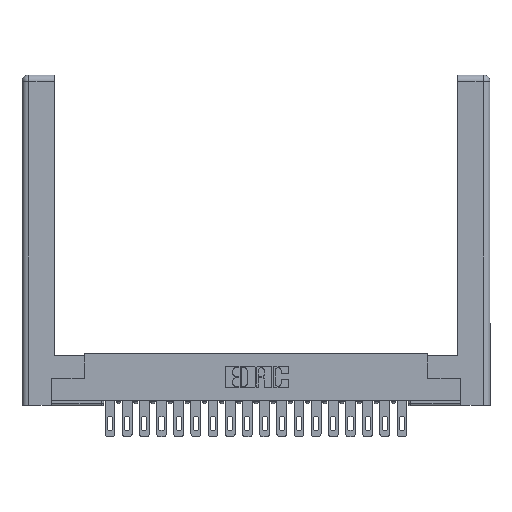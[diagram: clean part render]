
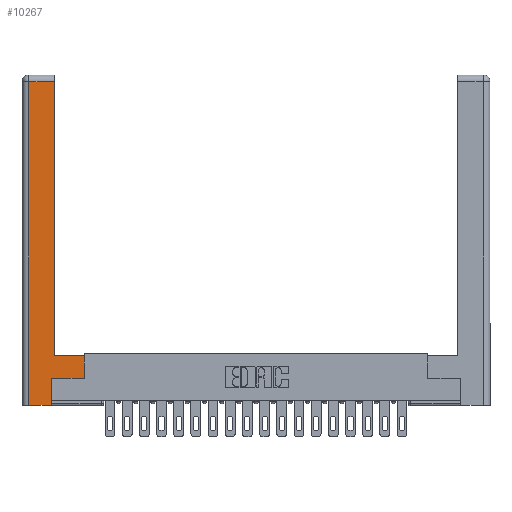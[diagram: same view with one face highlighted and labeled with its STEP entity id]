
A CAD part, top view. The second image highlights one B-rep face of the part: STEP entity #10267.
In plain terms, the highlighted planar face has unit normal (0, 0, 1).
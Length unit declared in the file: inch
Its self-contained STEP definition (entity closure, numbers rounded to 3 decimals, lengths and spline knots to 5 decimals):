
#67 = ORIENTED_EDGE ( 'NONE', *, *, #13105, .T. ) ;
#101 = ORIENTED_EDGE ( 'NONE', *, *, #14070, .T. ) ;
#666 = CARTESIAN_POINT ( 'NONE',  ( 0.565, 0.245, 0. ) ) ;
#947 = DIRECTION ( 'NONE',  ( 0., 1., 0. ) ) ;
#1088 = CARTESIAN_POINT ( 'NONE',  ( 0.265, 0.245, 0. ) ) ;
#1178 = VECTOR ( 'NONE', #18576, 39.37008 ) ;
#1301 = ORIENTED_EDGE ( 'NONE', *, *, #3292, .T. ) ;
#1410 = DIRECTION ( 'NONE',  ( 1., 0., 0. ) ) ;
#2432 = EDGE_CURVE ( 'NONE', #15426, #3903, #2820, .T. ) ;
#2820 = LINE ( 'NONE', #9255, #4693 ) ;
#3093 = PLANE ( 'NONE',  #21550 ) ;
#3292 = EDGE_CURVE ( 'NONE', #12812, #11096, #19490, .T. ) ;
#3414 = DIRECTION ( 'NONE',  ( -1., 0., 0. ) ) ;
#3785 = CARTESIAN_POINT ( 'NONE',  ( 0.565, 0.45, 0. ) ) ;
#3903 = VERTEX_POINT ( 'NONE', #18792 ) ;
#4213 = ORIENTED_EDGE ( 'NONE', *, *, #19601, .T. ) ;
#4693 = VECTOR ( 'NONE', #947, 39.37008 ) ;
#4699 = LINE ( 'NONE', #17998, #10013 ) ;
#4708 = VECTOR ( 'NONE', #21230, 39.37008 ) ;
#5031 = VECTOR ( 'NONE', #17765, 39.37008 ) ;
#5453 = DIRECTION ( 'NONE',  ( -1., 0., 0. ) ) ;
#6202 = VECTOR ( 'NONE', #12877, 39.37008 ) ;
#7429 = ORIENTED_EDGE ( 'NONE', *, *, #18138, .T. ) ;
#7685 = CARTESIAN_POINT ( 'NONE',  ( 0.0615, 0., 0. ) ) ;
#7697 = DIRECTION ( 'NONE',  ( 0., 1., 0. ) ) ;
#8512 = CARTESIAN_POINT ( 'NONE',  ( 0.0615, 2.94, 0. ) ) ;
#8569 = CARTESIAN_POINT ( 'NONE',  ( 0.0615, 0., 0. ) ) ;
#9255 = CARTESIAN_POINT ( 'NONE',  ( 0.295, 3., 0. ) ) ;
#9862 = CARTESIAN_POINT ( 'NONE',  ( 0.565, 0.45, 0. ) ) ;
#10013 = VECTOR ( 'NONE', #1410, 39.37008 ) ;
#10267 = ADVANCED_FACE ( 'NONE', ( #11577 ), #3093, .F. ) ;
#10383 = CARTESIAN_POINT ( 'NONE',  ( 0.265, 0., 0. ) ) ;
#10795 = EDGE_CURVE ( 'NONE', #20568, #20995, #4699, .T. ) ;
#10889 = CARTESIAN_POINT ( 'NONE',  ( 0.295, 0.45, 0. ) ) ;
#10947 = CARTESIAN_POINT ( 'NONE',  ( 0.565, 0.245, 0. ) ) ;
#11066 = EDGE_CURVE ( 'NONE', #11096, #15426, #19307, .T. ) ;
#11096 = VERTEX_POINT ( 'NONE', #3785 ) ;
#11476 = DIRECTION ( 'NONE',  ( 0., 0., -1. ) ) ;
#11577 = FACE_OUTER_BOUND ( 'NONE', #19947, .T. ) ;
#11805 = VECTOR ( 'NONE', #5453, 39.37008 ) ;
#12812 = VERTEX_POINT ( 'NONE', #10947 ) ;
#12877 = DIRECTION ( 'NONE',  ( 0., 1., 0. ) ) ;
#13105 = EDGE_CURVE ( 'NONE', #21238, #12812, #20766, .T. ) ;
#13149 = CARTESIAN_POINT ( 'NONE',  ( 0.0615, 2.94, 0. ) ) ;
#13505 = ORIENTED_EDGE ( 'NONE', *, *, #2432, .T. ) ;
#13707 = VERTEX_POINT ( 'NONE', #13149 ) ;
#14070 = EDGE_CURVE ( 'NONE', #13707, #20568, #16401, .T. ) ;
#14854 = CARTESIAN_POINT ( 'NONE',  ( 0., 0., 0. ) ) ;
#15426 = VERTEX_POINT ( 'NONE', #18996 ) ;
#15485 = LINE ( 'NONE', #8512, #11805 ) ;
#16401 = LINE ( 'NONE', #7685, #4708 ) ;
#17687 = LINE ( 'NONE', #1088, #6202 ) ;
#17765 = DIRECTION ( 'NONE',  ( -1., 0., 0. ) ) ;
#17998 = CARTESIAN_POINT ( 'NONE',  ( 0.265, 0., 0. ) ) ;
#18138 = EDGE_CURVE ( 'NONE', #20995, #21238, #17687, .T. ) ;
#18576 = DIRECTION ( 'NONE',  ( 1., 0., 0. ) ) ;
#18792 = CARTESIAN_POINT ( 'NONE',  ( 0.295, 2.94, 0. ) ) ;
#18996 = CARTESIAN_POINT ( 'NONE',  ( 0.295, 0.45, 0. ) ) ;
#19070 = VECTOR ( 'NONE', #7697, 39.37008 ) ;
#19307 = LINE ( 'NONE', #10889, #5031 ) ;
#19490 = LINE ( 'NONE', #9862, #19070 ) ;
#19601 = EDGE_CURVE ( 'NONE', #3903, #13707, #15485, .T. ) ;
#19735 = CARTESIAN_POINT ( 'NONE',  ( 0.265, 0.245, 0. ) ) ;
#19947 = EDGE_LOOP ( 'NONE', ( #13505, #4213, #101, #21081, #7429, #67, #1301, #21035 ) ) ;
#20568 = VERTEX_POINT ( 'NONE', #8569 ) ;
#20766 = LINE ( 'NONE', #666, #1178 ) ;
#20995 = VERTEX_POINT ( 'NONE', #10383 ) ;
#21035 = ORIENTED_EDGE ( 'NONE', *, *, #11066, .T. ) ;
#21081 = ORIENTED_EDGE ( 'NONE', *, *, #10795, .T. ) ;
#21230 = DIRECTION ( 'NONE',  ( 0., -1., 0. ) ) ;
#21238 = VERTEX_POINT ( 'NONE', #19735 ) ;
#21550 = AXIS2_PLACEMENT_3D ( 'NONE', #14854, #11476, #3414 ) ;
